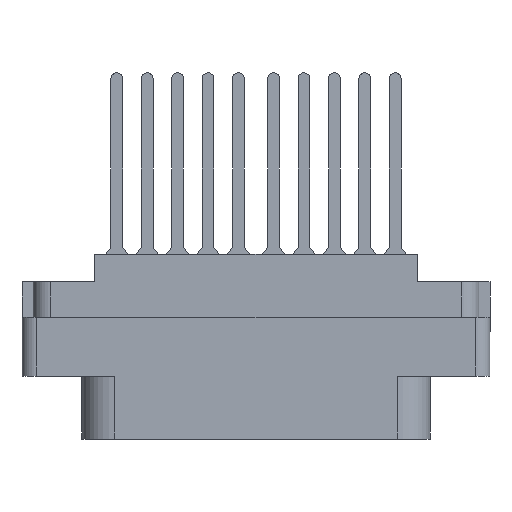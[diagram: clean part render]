
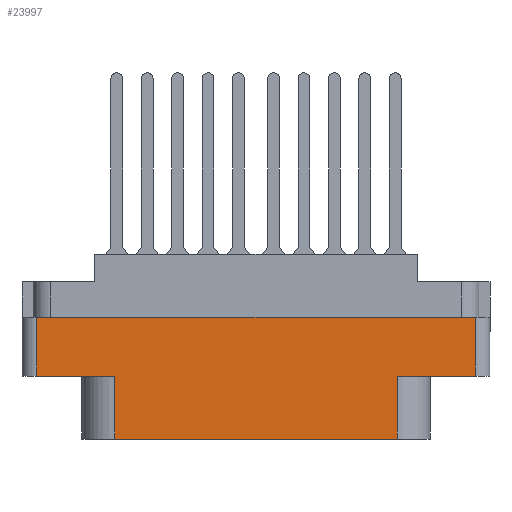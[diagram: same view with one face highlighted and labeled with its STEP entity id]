
A CAD part, front view. The second image highlights one B-rep face of the part: STEP entity #23997.
In plain terms, the highlighted planar face has unit normal (0, -1, 0).
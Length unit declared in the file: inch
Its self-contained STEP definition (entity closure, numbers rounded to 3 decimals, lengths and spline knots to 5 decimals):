
#71 = VECTOR ( 'NONE', #30955, 39.37008 ) ;
#108 = FACE_OUTER_BOUND ( 'NONE', #3949, .T. ) ;
#236 = DIRECTION ( 'NONE',  ( 0., 0., -1. ) ) ;
#1627 = ORIENTED_EDGE ( 'NONE', *, *, #30627, .T. ) ;
#2255 = ORIENTED_EDGE ( 'NONE', *, *, #12250, .T. ) ;
#3507 = LINE ( 'NONE', #25152, #22650 ) ;
#3559 = CARTESIAN_POINT ( 'NONE',  ( -0.604, -0.438, -0.52 ) ) ;
#3940 = CARTESIAN_POINT ( 'NONE',  ( -0.938, -0.438, -0.789 ) ) ;
#3949 = EDGE_LOOP ( 'NONE', ( #31812, #13198, #11496, #1627, #11701, #2255, #8638, #10991 ) ) ;
#3982 = EDGE_CURVE ( 'NONE', #10689, #17696, #8620, .T. ) ;
#4340 = VECTOR ( 'NONE', #33337, 39.37008 ) ;
#4369 = DIRECTION ( 'NONE',  ( -1., 0., 0. ) ) ;
#5082 = DIRECTION ( 'NONE',  ( 0., 0., 1. ) ) ;
#8620 = LINE ( 'NONE', #19142, #30975 ) ;
#8638 = ORIENTED_EDGE ( 'NONE', *, *, #21343, .F. ) ;
#8647 = LINE ( 'NONE', #3940, #30579 ) ;
#9899 = CARTESIAN_POINT ( 'NONE',  ( 0.938, -0.438, -0.789 ) ) ;
#10689 = VERTEX_POINT ( 'NONE', #27083 ) ;
#10839 = CARTESIAN_POINT ( 'NONE',  ( 0.938, -0.438, -0.52 ) ) ;
#10991 = ORIENTED_EDGE ( 'NONE', *, *, #12157, .T. ) ;
#11496 = ORIENTED_EDGE ( 'NONE', *, *, #3982, .T. ) ;
#11544 = DIRECTION ( 'NONE',  ( 1., 0., 0. ) ) ;
#11581 = DIRECTION ( 'NONE',  ( 0., 0., -1. ) ) ;
#11701 = ORIENTED_EDGE ( 'NONE', *, *, #24629, .T. ) ;
#11758 = EDGE_CURVE ( 'NONE', #15130, #31516, #21892, .T. ) ;
#11776 = PLANE ( 'NONE',  #12430 ) ;
#11887 = DIRECTION ( 'NONE',  ( 0., -1., 0. ) ) ;
#12157 = EDGE_CURVE ( 'NONE', #26921, #31516, #29570, .T. ) ;
#12250 = EDGE_CURVE ( 'NONE', #14372, #29104, #17824, .T. ) ;
#12430 = AXIS2_PLACEMENT_3D ( 'NONE', #29947, #11887, #17355 ) ;
#13198 = ORIENTED_EDGE ( 'NONE', *, *, #24721, .T. ) ;
#13770 = VECTOR ( 'NONE', #28531, 39.37008 ) ;
#14372 = VERTEX_POINT ( 'NONE', #32364 ) ;
#15130 = VERTEX_POINT ( 'NONE', #25680 ) ;
#16594 = CARTESIAN_POINT ( 'NONE',  ( -0.604, -0.438, -0.789 ) ) ;
#17355 = DIRECTION ( 'NONE',  ( 0., 0., -1. ) ) ;
#17696 = VERTEX_POINT ( 'NONE', #3559 ) ;
#17824 = LINE ( 'NONE', #18053, #21862 ) ;
#18010 = VECTOR ( 'NONE', #236, 39.37008 ) ;
#18053 = CARTESIAN_POINT ( 'NONE',  ( 0.604, -0.438, -0.52 ) ) ;
#19142 = CARTESIAN_POINT ( 'NONE',  ( 0., -0.438, -0.52 ) ) ;
#21065 = CARTESIAN_POINT ( 'NONE',  ( -0.604, -0.438, -0.789 ) ) ;
#21343 = EDGE_CURVE ( 'NONE', #26921, #29104, #3507, .T. ) ;
#21862 = VECTOR ( 'NONE', #5082, 39.37008 ) ;
#21892 = LINE ( 'NONE', #30929, #13770 ) ;
#22650 = VECTOR ( 'NONE', #4369, 39.37008 ) ;
#23878 = CARTESIAN_POINT ( 'NONE',  ( 0.938, -0.438, -0.268 ) ) ;
#23997 = ADVANCED_FACE ( 'NONE', ( #108 ), #11776, .T. ) ;
#24629 = EDGE_CURVE ( 'NONE', #25684, #14372, #29748, .T. ) ;
#24721 = EDGE_CURVE ( 'NONE', #15130, #10689, #8647, .T. ) ;
#25152 = CARTESIAN_POINT ( 'NONE',  ( 0., -0.438, -0.52 ) ) ;
#25359 = CARTESIAN_POINT ( 'NONE',  ( -1., -0.438, -0.789 ) ) ;
#25680 = CARTESIAN_POINT ( 'NONE',  ( -0.938, -0.438, -0.268 ) ) ;
#25684 = VERTEX_POINT ( 'NONE', #16594 ) ;
#26921 = VERTEX_POINT ( 'NONE', #10839 ) ;
#27083 = CARTESIAN_POINT ( 'NONE',  ( -0.938, -0.438, -0.52 ) ) ;
#28531 = DIRECTION ( 'NONE',  ( 1., 0., 0. ) ) ;
#29104 = VERTEX_POINT ( 'NONE', #30662 ) ;
#29570 = LINE ( 'NONE', #9899, #4340 ) ;
#29748 = LINE ( 'NONE', #25359, #71 ) ;
#29800 = LINE ( 'NONE', #21065, #18010 ) ;
#29947 = CARTESIAN_POINT ( 'NONE',  ( -1., -0.438, -0.789 ) ) ;
#30579 = VECTOR ( 'NONE', #11581, 39.37008 ) ;
#30627 = EDGE_CURVE ( 'NONE', #17696, #25684, #29800, .T. ) ;
#30662 = CARTESIAN_POINT ( 'NONE',  ( 0.604, -0.438, -0.52 ) ) ;
#30929 = CARTESIAN_POINT ( 'NONE',  ( 0., -0.438, -0.268 ) ) ;
#30955 = DIRECTION ( 'NONE',  ( 1., 0., 0. ) ) ;
#30975 = VECTOR ( 'NONE', #11544, 39.37008 ) ;
#31516 = VERTEX_POINT ( 'NONE', #23878 ) ;
#31812 = ORIENTED_EDGE ( 'NONE', *, *, #11758, .F. ) ;
#32364 = CARTESIAN_POINT ( 'NONE',  ( 0.604, -0.438, -0.789 ) ) ;
#33337 = DIRECTION ( 'NONE',  ( 0., 0., 1. ) ) ;
